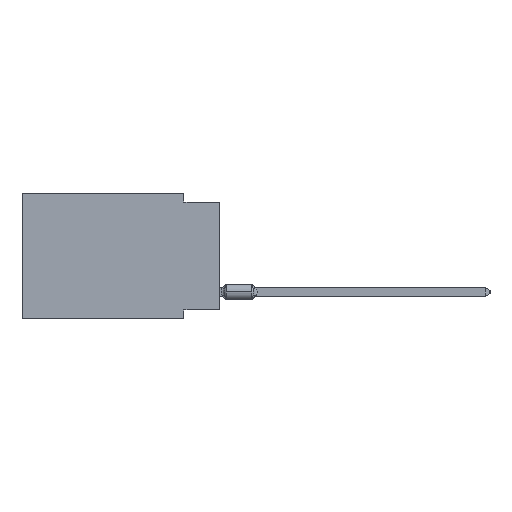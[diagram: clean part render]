
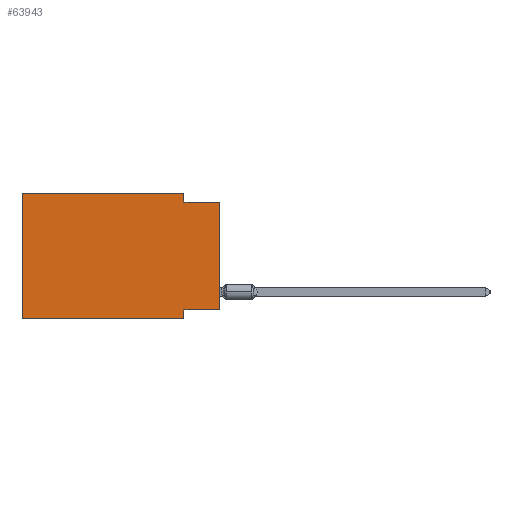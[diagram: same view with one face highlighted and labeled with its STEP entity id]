
A CAD part, left-side view. The second image highlights one B-rep face of the part: STEP entity #63943.
In plain terms, the highlighted planar face has unit normal (-1, 0, 0).
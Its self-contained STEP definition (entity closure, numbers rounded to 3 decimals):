
#451 = LINE ( 'NONE', #64238, #4389 ) ;
#564 = DIRECTION ( 'NONE',  ( 0., -1., 0. ) ) ;
#869 = EDGE_CURVE ( 'NONE', #3411, #33703, #12987, .T. ) ;
#1674 = ORIENTED_EDGE ( 'NONE', *, *, #63659, .T. ) ;
#2495 = VECTOR ( 'NONE', #48302, 1000. ) ;
#3312 = VECTOR ( 'NONE', #49224, 1000. ) ;
#3411 = VERTEX_POINT ( 'NONE', #57736 ) ;
#3924 = DIRECTION ( 'NONE',  ( 1., 0., 0. ) ) ;
#3940 = DIRECTION ( 'NONE',  ( 0., -1., 0. ) ) ;
#4389 = VECTOR ( 'NONE', #18337, 1000. ) ;
#5664 = EDGE_CURVE ( 'NONE', #54711, #17965, #25519, .T. ) ;
#7556 = CARTESIAN_POINT ( 'NONE',  ( 0., 2.54, -8.89 ) ) ;
#8243 = CARTESIAN_POINT ( 'NONE',  ( 0., 0., -8.255 ) ) ;
#8501 = VECTOR ( 'NONE', #564, 1000. ) ;
#10058 = CARTESIAN_POINT ( 'NONE',  ( 0., 2.54, -8.89 ) ) ;
#12987 = LINE ( 'NONE', #7556, #14897 ) ;
#14652 = EDGE_CURVE ( 'NONE', #31693, #3411, #47135, .T. ) ;
#14897 = VECTOR ( 'NONE', #18074, 1000. ) ;
#15013 = VERTEX_POINT ( 'NONE', #57567 ) ;
#15852 = ORIENTED_EDGE ( 'NONE', *, *, #14652, .F. ) ;
#16032 = CARTESIAN_POINT ( 'NONE',  ( 0., 13.97, 0. ) ) ;
#16686 = VECTOR ( 'NONE', #71229, 1000. ) ;
#16799 = AXIS2_PLACEMENT_3D ( 'NONE', #39299, #3924, #57944 ) ;
#17965 = VERTEX_POINT ( 'NONE', #16032 ) ;
#18074 = DIRECTION ( 'NONE',  ( 0., 0., -1. ) ) ;
#18337 = DIRECTION ( 'NONE',  ( 0., 0., 1. ) ) ;
#19907 = EDGE_LOOP ( 'NONE', ( #1674, #55495, #34445, #32132, #42557, #34841, #40577, #15852 ) ) ;
#22084 = VECTOR ( 'NONE', #3940, 1000. ) ;
#25519 = LINE ( 'NONE', #31732, #3312 ) ;
#28474 = VERTEX_POINT ( 'NONE', #55593 ) ;
#31693 = VERTEX_POINT ( 'NONE', #8243 ) ;
#31732 = CARTESIAN_POINT ( 'NONE',  ( 0., 13.97, 0. ) ) ;
#31858 = EDGE_CURVE ( 'NONE', #15013, #28474, #49074, .T. ) ;
#32132 = ORIENTED_EDGE ( 'NONE', *, *, #42497, .F. ) ;
#33658 = CARTESIAN_POINT ( 'NONE',  ( 0., 0., -8.255 ) ) ;
#33703 = VERTEX_POINT ( 'NONE', #10058 ) ;
#34237 = PLANE ( 'NONE',  #16799 ) ;
#34445 = ORIENTED_EDGE ( 'NONE', *, *, #31858, .F. ) ;
#34841 = ORIENTED_EDGE ( 'NONE', *, *, #47079, .T. ) ;
#35356 = VERTEX_POINT ( 'NONE', #64384 ) ;
#37067 = EDGE_CURVE ( 'NONE', #28474, #35356, #64094, .T. ) ;
#38533 = CARTESIAN_POINT ( 'NONE',  ( 0., 13.97, -8.89 ) ) ;
#38671 = CARTESIAN_POINT ( 'NONE',  ( 0., 13.97, -8.89 ) ) ;
#39299 = CARTESIAN_POINT ( 'NONE',  ( 0., 13.97, 0. ) ) ;
#40577 = ORIENTED_EDGE ( 'NONE', *, *, #869, .F. ) ;
#42497 = EDGE_CURVE ( 'NONE', #17965, #15013, #52294, .T. ) ;
#42557 = ORIENTED_EDGE ( 'NONE', *, *, #5664, .F. ) ;
#45099 = VECTOR ( 'NONE', #70316, 1000. ) ;
#47079 = EDGE_CURVE ( 'NONE', #54711, #33703, #56812, .T. ) ;
#47135 = LINE ( 'NONE', #33658, #16686 ) ;
#48302 = DIRECTION ( 'NONE',  ( 0., 0., -1. ) ) ;
#49074 = LINE ( 'NONE', #55290, #2495 ) ;
#49224 = DIRECTION ( 'NONE',  ( 0., 0., 1. ) ) ;
#52294 = LINE ( 'NONE', #76037, #8501 ) ;
#54711 = VERTEX_POINT ( 'NONE', #38671 ) ;
#55290 = CARTESIAN_POINT ( 'NONE',  ( 0., 2.54, 0. ) ) ;
#55495 = ORIENTED_EDGE ( 'NONE', *, *, #37067, .F. ) ;
#55593 = CARTESIAN_POINT ( 'NONE',  ( 0., 2.54, -0.635 ) ) ;
#56812 = LINE ( 'NONE', #38533, #22084 ) ;
#57567 = CARTESIAN_POINT ( 'NONE',  ( 0., 2.54, 0. ) ) ;
#57736 = CARTESIAN_POINT ( 'NONE',  ( 0., 2.54, -8.255 ) ) ;
#57944 = DIRECTION ( 'NONE',  ( 0., 0., -1. ) ) ;
#63659 = EDGE_CURVE ( 'NONE', #31693, #35356, #451, .T. ) ;
#63772 = FACE_OUTER_BOUND ( 'NONE', #19907, .T. ) ;
#63943 = ADVANCED_FACE ( 'NONE', ( #63772 ), #34237, .F. ) ;
#64094 = LINE ( 'NONE', #69927, #45099 ) ;
#64238 = CARTESIAN_POINT ( 'NONE',  ( 0., 0., 0. ) ) ;
#64384 = CARTESIAN_POINT ( 'NONE',  ( 0., 0., -0.635 ) ) ;
#69927 = CARTESIAN_POINT ( 'NONE',  ( 0., 0., -0.635 ) ) ;
#70316 = DIRECTION ( 'NONE',  ( 0., -1., 0. ) ) ;
#71229 = DIRECTION ( 'NONE',  ( 0., 1., 0. ) ) ;
#76037 = CARTESIAN_POINT ( 'NONE',  ( 0., 13.97, 0. ) ) ;
